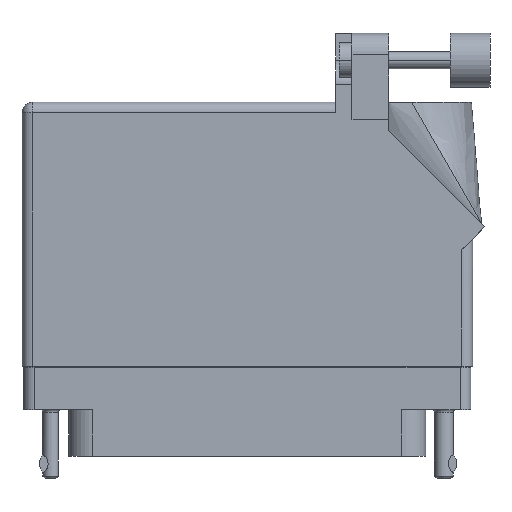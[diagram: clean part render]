
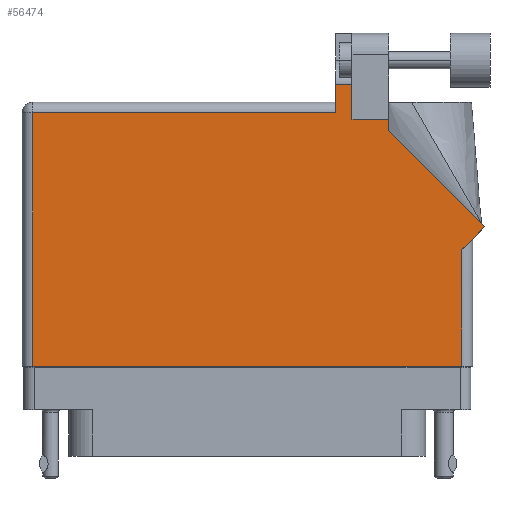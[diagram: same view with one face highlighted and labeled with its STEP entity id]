
A CAD part, front view. The second image highlights one B-rep face of the part: STEP entity #56474.
In plain terms, the highlighted face is planar.
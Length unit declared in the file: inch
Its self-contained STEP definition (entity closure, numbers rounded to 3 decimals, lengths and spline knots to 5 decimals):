
#311 = FACE_OUTER_BOUND ( 'NONE', #16548, .T. ) ;
#956 = VECTOR ( 'NONE', #56049, 39.37008 ) ;
#1302 = VERTEX_POINT ( 'NONE', #16968 ) ;
#1923 = ORIENTED_EDGE ( 'NONE', *, *, #30484, .T. ) ;
#2336 = CARTESIAN_POINT ( 'NONE',  ( 0.82, 1.33, 0.455 ) ) ;
#3720 = CARTESIAN_POINT ( 'NONE',  ( 0.513, 1.5315, 0.455 ) ) ;
#4993 = VERTEX_POINT ( 'NONE', #23803 ) ;
#5057 = VECTOR ( 'NONE', #26006, 39.37008 ) ;
#6114 = VECTOR ( 'NONE', #21243, 39.37008 ) ;
#6760 = LINE ( 'NONE', #12685, #12102 ) ;
#6904 = CARTESIAN_POINT ( 'NONE',  ( 0.513, 1.43, 0.455 ) ) ;
#7189 = VERTEX_POINT ( 'NONE', #58418 ) ;
#7219 = CARTESIAN_POINT ( 'NONE',  ( 1.37671, 0.70771, 0.455 ) ) ;
#7787 = LINE ( 'NONE', #26786, #41042 ) ;
#8251 = DIRECTION ( 'NONE',  ( 0., 1., 0. ) ) ;
#9392 = LINE ( 'NONE', #28391, #42761 ) ;
#12102 = VECTOR ( 'NONE', #12379, 39.37008 ) ;
#12379 = DIRECTION ( 'NONE',  ( 0., 1., 0. ) ) ;
#12680 = EDGE_CURVE ( 'NONE', #1302, #21934, #16999, .T. ) ;
#12685 = CARTESIAN_POINT ( 'NONE',  ( 0.607, 1.33, 0.455 ) ) ;
#13356 = VERTEX_POINT ( 'NONE', #59776 ) ;
#13521 = EDGE_CURVE ( 'NONE', #7189, #14502, #9392, .T. ) ;
#13750 = DIRECTION ( 'NONE',  ( -1., 0., 0. ) ) ;
#14102 = CARTESIAN_POINT ( 'NONE',  ( 0.82, 1.26442, 0.455 ) ) ;
#14350 = PLANE ( 'NONE',  #18507 ) ;
#14356 = CARTESIAN_POINT ( 'NONE',  ( 0.93777, 1.5315, 0.455 ) ) ;
#14502 = VERTEX_POINT ( 'NONE', #54966 ) ;
#16548 = EDGE_LOOP ( 'NONE', ( #52153, #1923, #29565, #54161, #58969, #49651, #26824, #22220, #38817, #35159, #40570 ) ) ;
#16968 = CARTESIAN_POINT ( 'NONE',  ( 0.82, 1.33, 0.455 ) ) ;
#16999 = LINE ( 'NONE', #2336, #5057 ) ;
#17483 = EDGE_CURVE ( 'NONE', #41337, #1302, #23441, .T. ) ;
#18056 = DIRECTION ( 'NONE',  ( 0.707, 0.707, 0. ) ) ;
#18507 = AXIS2_PLACEMENT_3D ( 'NONE', #23685, #56907, #47910 ) ;
#21243 = DIRECTION ( 'NONE',  ( 0., -1., 0. ) ) ;
#21934 = VERTEX_POINT ( 'NONE', #26259 ) ;
#22078 = LINE ( 'NONE', #46004, #24419 ) ;
#22220 = ORIENTED_EDGE ( 'NONE', *, *, #56756, .T. ) ;
#23441 = LINE ( 'NONE', #14102, #956 ) ;
#23685 = CARTESIAN_POINT ( 'NONE',  ( -1.306, 1.43, 0.455 ) ) ;
#23803 = CARTESIAN_POINT ( 'NONE',  ( 1.244, 0.575, 0.455 ) ) ;
#24419 = VECTOR ( 'NONE', #18056, 39.37008 ) ;
#25826 = CARTESIAN_POINT ( 'NONE',  ( 0.82, 1.26442, 0.455 ) ) ;
#26006 = DIRECTION ( 'NONE',  ( -1., 0., 0. ) ) ;
#26259 = CARTESIAN_POINT ( 'NONE',  ( 0.607, 1.33, 0.455 ) ) ;
#26786 = CARTESIAN_POINT ( 'NONE',  ( -1.244, -0.1, 0.455 ) ) ;
#26824 = ORIENTED_EDGE ( 'NONE', *, *, #35570, .T. ) ;
#28090 = CARTESIAN_POINT ( 'NONE',  ( -1.244, 1.368, 0.455 ) ) ;
#28304 = VERTEX_POINT ( 'NONE', #28090 ) ;
#28391 = CARTESIAN_POINT ( 'NONE',  ( -1.306, -0.1, 0.455 ) ) ;
#28763 = EDGE_CURVE ( 'NONE', #28304, #7189, #7787, .T. ) ;
#29565 = ORIENTED_EDGE ( 'NONE', *, *, #51972, .T. ) ;
#30045 = VERTEX_POINT ( 'NONE', #7219 ) ;
#30484 = EDGE_CURVE ( 'NONE', #13356, #32693, #33933, .T. ) ;
#31286 = LINE ( 'NONE', #59231, #31706 ) ;
#31706 = VECTOR ( 'NONE', #8251, 39.37008 ) ;
#31904 = EDGE_CURVE ( 'NONE', #30045, #41337, #47468, .T. ) ;
#32009 = VECTOR ( 'NONE', #42954, 39.37008 ) ;
#32693 = VERTEX_POINT ( 'NONE', #3720 ) ;
#33796 = CARTESIAN_POINT ( 'NONE',  ( 1.37671, 0.70771, 0.455 ) ) ;
#33849 = CARTESIAN_POINT ( 'NONE',  ( 0.513, 1.368, 0.455 ) ) ;
#33933 = LINE ( 'NONE', #14356, #32009 ) ;
#35159 = ORIENTED_EDGE ( 'NONE', *, *, #17483, .T. ) ;
#35570 = EDGE_CURVE ( 'NONE', #14502, #4993, #31286, .T. ) ;
#37388 = LINE ( 'NONE', #56302, #37499 ) ;
#37499 = VECTOR ( 'NONE', #13750, 39.37008 ) ;
#38817 = ORIENTED_EDGE ( 'NONE', *, *, #31904, .T. ) ;
#40570 = ORIENTED_EDGE ( 'NONE', *, *, #12680, .T. ) ;
#41042 = VECTOR ( 'NONE', #45740, 39.37008 ) ;
#41128 = LINE ( 'NONE', #6904, #6114 ) ;
#41337 = VERTEX_POINT ( 'NONE', #25826 ) ;
#41764 = VERTEX_POINT ( 'NONE', #33849 ) ;
#42761 = VECTOR ( 'NONE', #47329, 39.37008 ) ;
#42954 = DIRECTION ( 'NONE',  ( -1., 0., 0. ) ) ;
#43038 = EDGE_CURVE ( 'NONE', #41764, #28304, #37388, .T. ) ;
#43423 = DIRECTION ( 'NONE',  ( -0.707, 0.707, 0. ) ) ;
#45740 = DIRECTION ( 'NONE',  ( 0., -1., 0. ) ) ;
#46004 = CARTESIAN_POINT ( 'NONE',  ( 1.306, 0.637, 0.455 ) ) ;
#47329 = DIRECTION ( 'NONE',  ( 1., 0., 0. ) ) ;
#47468 = LINE ( 'NONE', #33796, #59933 ) ;
#47669 = EDGE_CURVE ( 'NONE', #21934, #13356, #6760, .T. ) ;
#47910 = DIRECTION ( 'NONE',  ( -1., 0., 0. ) ) ;
#49651 = ORIENTED_EDGE ( 'NONE', *, *, #13521, .T. ) ;
#51972 = EDGE_CURVE ( 'NONE', #32693, #41764, #41128, .T. ) ;
#52153 = ORIENTED_EDGE ( 'NONE', *, *, #47669, .T. ) ;
#54161 = ORIENTED_EDGE ( 'NONE', *, *, #43038, .T. ) ;
#54966 = CARTESIAN_POINT ( 'NONE',  ( 1.244, -0.1, 0.455 ) ) ;
#56049 = DIRECTION ( 'NONE',  ( 0., 1., 0. ) ) ;
#56302 = CARTESIAN_POINT ( 'NONE',  ( -1.306, 1.368, 0.455 ) ) ;
#56474 = ADVANCED_FACE ( 'NONE', ( #311 ), #14350, .F. ) ;
#56756 = EDGE_CURVE ( 'NONE', #4993, #30045, #22078, .T. ) ;
#56907 = DIRECTION ( 'NONE',  ( 0., 0., -1. ) ) ;
#58418 = CARTESIAN_POINT ( 'NONE',  ( -1.244, -0.1, 0.455 ) ) ;
#58969 = ORIENTED_EDGE ( 'NONE', *, *, #28763, .T. ) ;
#59231 = CARTESIAN_POINT ( 'NONE',  ( 1.244, 0.637, 0.455 ) ) ;
#59776 = CARTESIAN_POINT ( 'NONE',  ( 0.607, 1.5315, 0.455 ) ) ;
#59933 = VECTOR ( 'NONE', #43423, 39.37008 ) ;
